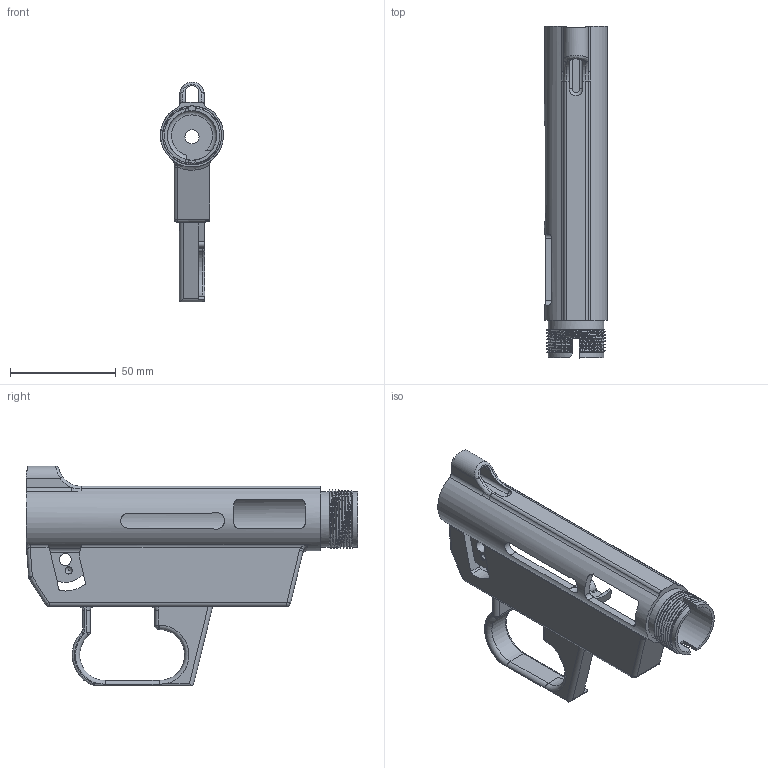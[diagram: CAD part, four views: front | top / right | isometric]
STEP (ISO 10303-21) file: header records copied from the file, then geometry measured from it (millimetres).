
FILE_DESCRIPTION(/* description */ (''),/* implementation_level */ '2;1');
FILE_NAME(/* name */ 'AR-7 Reciever for 3D Printing v8.step',/* time_stamp */ '2020-12-07T22:02:30-05:00',/* author */ (''),/* organization */ (''),/* preprocessor_version */ 'ST-DEVELOPER v18.1',/* originating_system */ 'Autodesk Translation Framework v9.3.0.1241',/* authorisation */ '');
FILE_SCHEMA (('AUTOMOTIVE_DESIGN { 1 0 10303 214 3 1 1 }'));
Length unit declared in the file: millimetre
Products named in the file (1): AR-7 Reciever for 3D Printing
Bounding box: 29.82 x 156.95 x 103.93 mm (x, y, z)
Volume: 58216 mm3; surface area: 40203.5 mm2
Topology: 1 solids, 1 shells, 338 faces, 940 edges, 600 vertices
Faces by surface type: cylinder 140, plane 135, bspline 37, torus 19, sphere 4, cone 3
Full cylindrical faces by diameter (mm): 3.45 x1, 3.75 x2, 3.95 x1, 4.3 x1, 5.02 x1, 5.65 x1, 6.65 x1, 7.75 x1, 23.4 x1, 26.132 x2, 26.3 x1, 27.85 x3
Entity records: 13906 total; most frequent: CARTESIAN_POINT 5381, ORIENTED_EDGE 1876, DIRECTION 1680, EDGE_CURVE 938, VERTEX_POINT 600, AXIS2_PLACEMENT_3D 600, LINE 480, VECTOR 480
